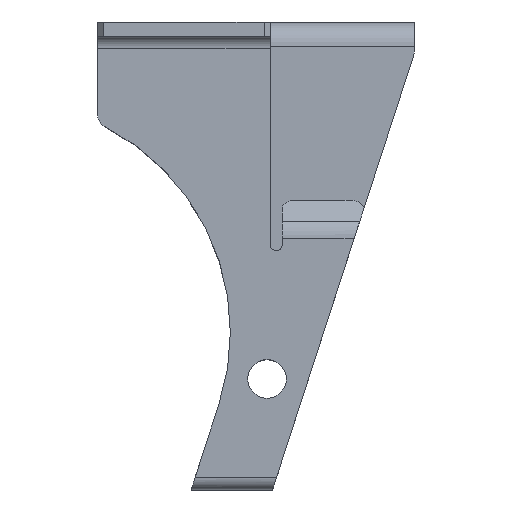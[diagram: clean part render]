
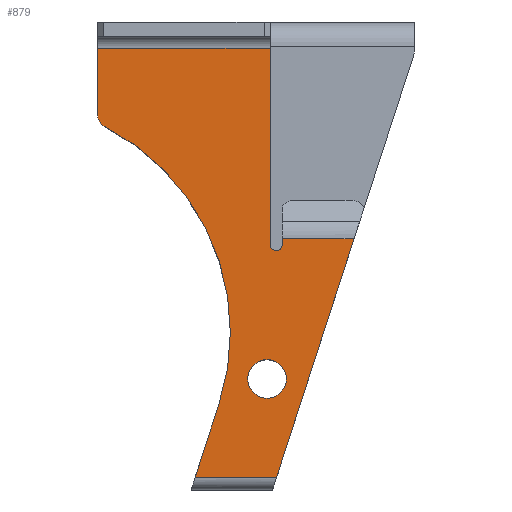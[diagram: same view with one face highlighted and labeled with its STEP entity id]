
A CAD part, top view. The second image highlights one B-rep face of the part: STEP entity #879.
In plain terms, the highlighted planar face has unit normal (0, 0, 1).
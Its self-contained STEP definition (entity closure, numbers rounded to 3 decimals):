
#16=FACE_BOUND('',#109,.T.);
#61=FACE_OUTER_BOUND('',#108,.T.);
#108=EDGE_LOOP('',(#635,#636,#637,#638,#639,#640,#641,#642,#643,#644,#645));
#109=EDGE_LOOP('',(#646));
#150=CIRCLE('',#940,0.5);
#156=CIRCLE('',#959,1.);
#157=CIRCLE('',#960,19.125);
#158=CIRCLE('',#961,1.6);
#175=LINE('',#1291,#267);
#198=LINE('',#1361,#290);
#199=LINE('',#1365,#291);
#200=LINE('',#1367,#292);
#201=LINE('',#1369,#293);
#202=LINE('',#1375,#294);
#203=LINE('',#1377,#295);
#204=LINE('',#1378,#296);
#267=VECTOR('',#1025,10.);
#290=VECTOR('',#1090,10.);
#291=VECTOR('',#1095,10.);
#292=VECTOR('',#1096,10.);
#293=VECTOR('',#1097,10.);
#294=VECTOR('',#1102,10.);
#295=VECTOR('',#1103,10.);
#296=VECTOR('',#1104,10.);
#359=VERTEX_POINT('',#1289);
#360=VERTEX_POINT('',#1290);
#368=VERTEX_POINT('',#1308);
#386=VERTEX_POINT('',#1360);
#387=VERTEX_POINT('',#1364);
#388=VERTEX_POINT('',#1366);
#389=VERTEX_POINT('',#1368);
#390=VERTEX_POINT('',#1370);
#391=VERTEX_POINT('',#1372);
#392=VERTEX_POINT('',#1374);
#393=VERTEX_POINT('',#1376);
#394=VERTEX_POINT('',#1379);
#447=EDGE_CURVE('',#359,#360,#175,.T.);
#457=EDGE_CURVE('',#368,#360,#150,.T.);
#482=EDGE_CURVE('',#359,#386,#198,.T.);
#484=EDGE_CURVE('',#368,#387,#199,.T.);
#485=EDGE_CURVE('',#388,#387,#200,.T.);
#486=EDGE_CURVE('',#388,#389,#201,.T.);
#487=EDGE_CURVE('',#390,#389,#156,.T.);
#488=EDGE_CURVE('',#390,#391,#157,.F.);
#489=EDGE_CURVE('',#391,#392,#202,.F.);
#490=EDGE_CURVE('',#393,#392,#203,.T.);
#491=EDGE_CURVE('',#393,#386,#204,.F.);
#492=EDGE_CURVE('',#394,#394,#158,.T.);
#635=ORIENTED_EDGE('',*,*,#447,.T.);
#636=ORIENTED_EDGE('',*,*,#457,.F.);
#637=ORIENTED_EDGE('',*,*,#484,.T.);
#638=ORIENTED_EDGE('',*,*,#485,.F.);
#639=ORIENTED_EDGE('',*,*,#486,.T.);
#640=ORIENTED_EDGE('',*,*,#487,.F.);
#641=ORIENTED_EDGE('',*,*,#488,.T.);
#642=ORIENTED_EDGE('',*,*,#489,.T.);
#643=ORIENTED_EDGE('',*,*,#490,.F.);
#644=ORIENTED_EDGE('',*,*,#491,.T.);
#645=ORIENTED_EDGE('',*,*,#482,.F.);
#646=ORIENTED_EDGE('',*,*,#492,.T.);
#848=PLANE('',#958);
#879=ADVANCED_FACE('',(#61,#16),#848,.T.);
#940=AXIS2_PLACEMENT_3D('',#1310,#1040,#1041);
#958=AXIS2_PLACEMENT_3D('',#1363,#1093,#1094);
#959=AXIS2_PLACEMENT_3D('',#1371,#1098,#1099);
#960=AXIS2_PLACEMENT_3D('',#1373,#1100,#1101);
#961=AXIS2_PLACEMENT_3D('',#1380,#1105,#1106);
#1025=DIRECTION('',(0.,-1.,0.));
#1040=DIRECTION('center_axis',(0.,0.,1.));
#1041=DIRECTION('ref_axis',(-0.707,-0.707,0.));
#1090=DIRECTION('',(1.,0.,0.));
#1093=DIRECTION('center_axis',(0.,0.,1.));
#1094=DIRECTION('ref_axis',(1.,0.,0.));
#1095=DIRECTION('',(0.,1.,0.));
#1096=DIRECTION('',(1.,0.,0.));
#1097=DIRECTION('',(0.,-1.,0.));
#1098=DIRECTION('center_axis',(0.,0.,-1.));
#1099=DIRECTION('ref_axis',(-0.853,-0.522,0.));
#1100=DIRECTION('center_axis',(0.,0.,1.));
#1101=DIRECTION('ref_axis',(0.951,-0.309,0.));
#1102=DIRECTION('',(0.309,0.951,0.));
#1103=DIRECTION('',(-1.,0.,0.));
#1104=DIRECTION('',(-0.309,-0.951,0.));
#1105=DIRECTION('center_axis',(0.,0.,-1.));
#1106=DIRECTION('ref_axis',(1.,0.,0.));
#1289=CARTESIAN_POINT('',(21.,-16.398,8.66));
#1290=CARTESIAN_POINT('',(21.,-16.898,8.66));
#1291=CARTESIAN_POINT('',(21.,-15.075,8.66));
#1308=CARTESIAN_POINT('',(20.,-16.898,8.66));
#1310=CARTESIAN_POINT('Origin',(20.5,-16.898,8.66));
#1360=CARTESIAN_POINT('',(26.948,-16.398,8.66));
#1361=CARTESIAN_POINT('',(18.542,-16.398,8.66));
#1363=CARTESIAN_POINT('Origin',(17.085,-17.75,8.66));
#1364=CARTESIAN_POINT('',(20.,-0.66,8.66));
#1365=CARTESIAN_POINT('',(20.,-18.993,8.66));
#1366=CARTESIAN_POINT('',(5.75,-0.66,8.66));
#1367=CARTESIAN_POINT('',(11.417,-0.66,8.66));
#1368=CARTESIAN_POINT('',(5.75,-6.225,8.66));
#1369=CARTESIAN_POINT('',(5.75,-8.125,8.66));
#1370=CARTESIAN_POINT('',(6.295,-7.116,8.66));
#1371=CARTESIAN_POINT('Origin',(6.75,-6.225,8.66));
#1372=CARTESIAN_POINT('',(15.781,-30.055,8.66));
#1373=CARTESIAN_POINT('Origin',(-2.408,-24.146,8.66));
#1374=CARTESIAN_POINT('',(13.797,-36.16,8.66));
#1375=CARTESIAN_POINT('',(16.435,-28.04,8.66));
#1376=CARTESIAN_POINT('',(20.527,-36.16,8.66));
#1377=CARTESIAN_POINT('',(18.654,-36.16,8.66));
#1378=CARTESIAN_POINT('',(28.705,-10.99,8.66));
#1379=CARTESIAN_POINT('',(18.15,-28.,8.66));
#1380=CARTESIAN_POINT('Origin',(19.75,-28.,8.66));
